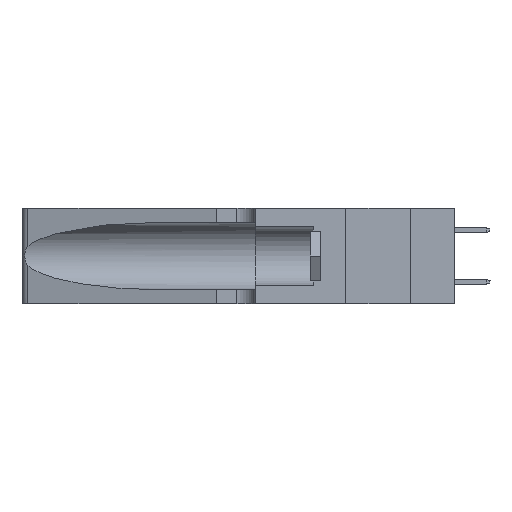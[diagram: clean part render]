
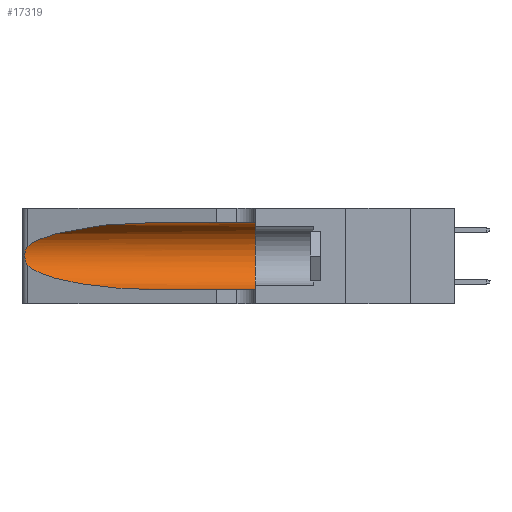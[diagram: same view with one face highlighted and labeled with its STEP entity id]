
A CAD part, left-side view. The second image highlights one B-rep face of the part: STEP entity #17319.
In plain terms, the highlighted cylindrical face has radius 3.308 mm (diameter 6.617 mm), a partial arc.
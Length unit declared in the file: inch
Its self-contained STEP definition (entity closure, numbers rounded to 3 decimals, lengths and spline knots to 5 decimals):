
#212 = DIRECTION ( 'NONE',  ( 0., 1., 0. ) ) ;
#249 = VERTEX_POINT ( 'NONE', #25840 ) ;
#387 = VERTEX_POINT ( 'NONE', #26606 ) ;
#716 = CARTESIAN_POINT ( 'NONE',  ( 0.1305, 0.35, 0.05475 ) ) ;
#901 = DIRECTION ( 'NONE',  ( 0., -1., 0. ) ) ;
#2689 = CARTESIAN_POINT ( 'NONE',  ( 0.25555, 1.22993, 0.14849 ) ) ;
#2880 = ORIENTED_EDGE ( 'NONE', *, *, #29462, .F. ) ;
#2938 = CARTESIAN_POINT ( 'NONE',  ( 0.1305, 0.35, 0.185 ) ) ;
#4996 = EDGE_LOOP ( 'NONE', ( #13318, #27295, #21330, #26557, #19040, #2880 ) ) ;
#5360 = DIRECTION ( 'NONE',  ( 0., -1., 0. ) ) ;
#5495 = DIRECTION ( 'NONE',  ( 0., 0., 1. ) ) ;
#5959 = EDGE_CURVE ( 'NONE', #249, #17579, #10582, .T. ) ;
#6278 = VERTEX_POINT ( 'NONE', #8714 ) ;
#6930 = VERTEX_POINT ( 'NONE', #19770 ) ;
#7565 = CARTESIAN_POINT ( 'NONE',  ( 0.1305, 1.61858, 0.185 ) ) ;
#7583 = CARTESIAN_POINT ( 'NONE',  ( 0.18966, 0.96281, 0.31525 ) ) ;
#7618 = LINE ( 'NONE', #15117, #19423 ) ;
#8246 = CARTESIAN_POINT ( 'NONE',  ( 0.26017, 1.23833, 0.17102 ) ) ;
#8369 = CARTESIAN_POINT ( 'NONE',  ( 0.1305, 1.61858, 0.05475 ) ) ;
#8714 = CARTESIAN_POINT ( 'NONE',  ( 0.1305, 0.72297, 0.31525 ) ) ;
#8855 = CARTESIAN_POINT ( 'NONE',  ( 0.2373, 1.15595, 0.08982 ) ) ;
#9699 = B_SPLINE_CURVE_WITH_KNOTS ( 'NONE', 3,
 ( #14947, #12861, #22576, #10612, #24641, #12555, #20344, #22266, #8246, #27666, #14780, #24475, #2689, #22108 ),
 .UNSPECIFIED., .F., .F.,
 ( 4, 2, 2, 2, 2, 2, 4 ),
 ( 0., 0.00027, 0.00053, 0.00107, 0.0016, 0.00187, 0.00214 ),
 .UNSPECIFIED. ) ;
#10249 = DIRECTION ( 'NONE',  ( 0., 0., -1. ) ) ;
#10420 = CARTESIAN_POINT ( 'NONE',  ( 0.25487, 1.22718, 0.22369 ) ) ;
#10582 = LINE ( 'NONE', #8369, #27047 ) ;
#10612 = CARTESIAN_POINT ( 'NONE',  ( 0.25787, 1.23484, 0.2124 ) ) ;
#12463 = EDGE_CURVE ( 'NONE', #6278, #28103, #17732, .T. ) ;
#12555 = CARTESIAN_POINT ( 'NONE',  ( 0.26018, 1.23835, 0.19895 ) ) ;
#12706 = DIRECTION ( 'NONE',  ( 0., -1., 0. ) ) ;
#12728 = AXIS2_PLACEMENT_3D ( 'NONE', #7565, #5360, #10249 ) ;
#12861 = CARTESIAN_POINT ( 'NONE',  ( 0.25555, 1.22994, 0.2215 ) ) ;
#13318 = ORIENTED_EDGE ( 'NONE', *, *, #12463, .T. ) ;
#13969 = CIRCLE ( 'NONE', #19598, 0.13025 ) ;
#14780 = CARTESIAN_POINT ( 'NONE',  ( 0.25789, 1.23486, 0.15765 ) ) ;
#14947 = CARTESIAN_POINT ( 'NONE',  ( 0.25487, 1.22718, 0.22369 ) ) ;
#15117 = CARTESIAN_POINT ( 'NONE',  ( 0.1305, 1.61858, 0.31525 ) ) ;
#17319 = ADVANCED_FACE ( 'NONE', ( #24266 ), #22050, .F. ) ;
#17579 = VERTEX_POINT ( 'NONE', #716 ) ;
#17732 =( BOUNDED_CURVE ( )  B_SPLINE_CURVE ( 3, ( #29400, #7583, #29554, #19844 ),
 .UNSPECIFIED., .F., .T. ) 
 B_SPLINE_CURVE_WITH_KNOTS ( ( 4, 4 ),
 ( 1.5708, 2.84003 ),
 .UNSPECIFIED. ) 
 CURVE ( )  GEOMETRIC_REPRESENTATION_ITEM ( )  RATIONAL_B_SPLINE_CURVE ( ( 1., 0.87, 0.87, 1. ) ) 
 REPRESENTATION_ITEM ( '' )  );
#18756 =( BOUNDED_CURVE ( )  B_SPLINE_CURVE ( 3, ( #25417, #8855, #30671, #20671 ),
 .UNSPECIFIED., .F., .T. ) 
 B_SPLINE_CURVE_WITH_KNOTS ( ( 4, 4 ),
 ( 3.44316, 4.71239 ),
 .UNSPECIFIED. ) 
 CURVE ( )  GEOMETRIC_REPRESENTATION_ITEM ( )  RATIONAL_B_SPLINE_CURVE ( ( 1., 0.87, 0.87, 1. ) ) 
 REPRESENTATION_ITEM ( '' )  );
#19040 = ORIENTED_EDGE ( 'NONE', *, *, #26213, .F. ) ;
#19423 = VECTOR ( 'NONE', #12706, 39.37008 ) ;
#19598 = AXIS2_PLACEMENT_3D ( 'NONE', #2938, #212, #5495 ) ;
#19770 = CARTESIAN_POINT ( 'NONE',  ( 0.1305, 0.35, 0.31525 ) ) ;
#19844 = CARTESIAN_POINT ( 'NONE',  ( 0.25487, 1.22718, 0.22369 ) ) ;
#20344 = CARTESIAN_POINT ( 'NONE',  ( 0.26075, 1.23896, 0.19203 ) ) ;
#20671 = CARTESIAN_POINT ( 'NONE',  ( 0.1305, 0.72297, 0.05475 ) ) ;
#21330 = ORIENTED_EDGE ( 'NONE', *, *, #25518, .T. ) ;
#22050 = CYLINDRICAL_SURFACE ( 'NONE', #12728, 0.13025 ) ;
#22108 = CARTESIAN_POINT ( 'NONE',  ( 0.25487, 1.22718, 0.14631 ) ) ;
#22266 = CARTESIAN_POINT ( 'NONE',  ( 0.26075, 1.23896, 0.178 ) ) ;
#22576 = CARTESIAN_POINT ( 'NONE',  ( 0.25639, 1.23184, 0.21858 ) ) ;
#24266 = FACE_OUTER_BOUND ( 'NONE', #4996, .T. ) ;
#24475 = CARTESIAN_POINT ( 'NONE',  ( 0.25639, 1.23186, 0.15144 ) ) ;
#24641 = CARTESIAN_POINT ( 'NONE',  ( 0.25854, 1.2359, 0.20912 ) ) ;
#25417 = CARTESIAN_POINT ( 'NONE',  ( 0.25487, 1.22718, 0.14631 ) ) ;
#25426 = EDGE_CURVE ( 'NONE', #28103, #387, #9699, .T. ) ;
#25518 = EDGE_CURVE ( 'NONE', #387, #249, #18756, .T. ) ;
#25840 = CARTESIAN_POINT ( 'NONE',  ( 0.1305, 0.72297, 0.05475 ) ) ;
#26213 = EDGE_CURVE ( 'NONE', #6930, #17579, #13969, .T. ) ;
#26557 = ORIENTED_EDGE ( 'NONE', *, *, #5959, .T. ) ;
#26606 = CARTESIAN_POINT ( 'NONE',  ( 0.25487, 1.22718, 0.14631 ) ) ;
#27047 = VECTOR ( 'NONE', #901, 39.37008 ) ;
#27295 = ORIENTED_EDGE ( 'NONE', *, *, #25426, .T. ) ;
#27666 = CARTESIAN_POINT ( 'NONE',  ( 0.25856, 1.23593, 0.16098 ) ) ;
#28103 = VERTEX_POINT ( 'NONE', #10420 ) ;
#29400 = CARTESIAN_POINT ( 'NONE',  ( 0.1305, 0.72297, 0.31525 ) ) ;
#29462 = EDGE_CURVE ( 'NONE', #6278, #6930, #7618, .T. ) ;
#29554 = CARTESIAN_POINT ( 'NONE',  ( 0.2373, 1.15595, 0.28018 ) ) ;
#30671 = CARTESIAN_POINT ( 'NONE',  ( 0.18966, 0.96281, 0.05475 ) ) ;
